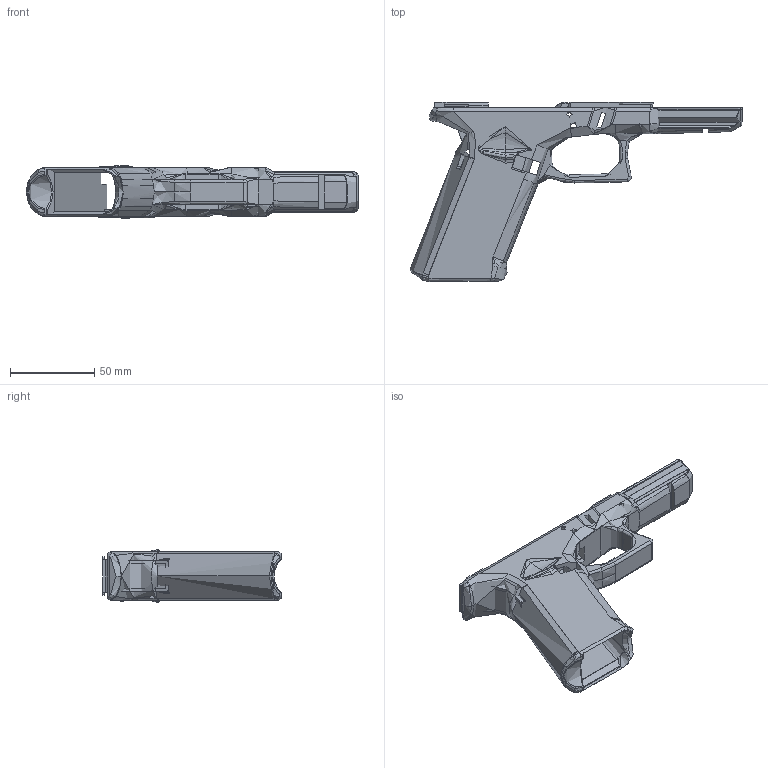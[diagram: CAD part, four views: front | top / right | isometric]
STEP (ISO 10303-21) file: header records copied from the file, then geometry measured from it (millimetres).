
FILE_DESCRIPTION(/* description */ (''),/* implementation_level */ '2;1');
FILE_NAME(/* name */ 'G17 P80 Rails.step',/* time_stamp */ '2019-09-29T13:28:27-04:00',/* author */ (''),/* organization */ (''),/* preprocessor_version */ 'ST-DEVELOPER v18',/* originating_system */ 'Autodesk Translation Framework v8.6.0.1094',/* authorisation */ '');
FILE_SCHEMA (('AUTOMOTIVE_DESIGN { 1 0 10303 214 3 1 1 }'));
Products named in the file (3): G17 P80 Rails; P80 Front Rails; P80 Rear Rails
Assembly tree (2 placements, depth 2):
  G17 P80 Rails
    P80 Front Rails
    P80 Rear Rails
Bounding box: 197.56 x 106.5 x 31.38 mm (x, y, z)
Volume: 94360.8 mm3
Topology: 3 solids, 7 shells, 878 faces, 2410 edges, 1509 vertices
Faces by surface type: bspline 382, plane 263, cylinder 183, torus 21, cone 19, sphere 10
Full cylindrical faces by diameter (mm): 3 x5, 3.2 x4, 3.5 x2, 3.8 x4
Entity records: 69030 total; most frequent: CARTESIAN_POINT 49261, ORIENTED_EDGE 4782, DIRECTION 3211, EDGE_CURVE 2391, VERTEX_POINT 1510, AXIS2_PLACEMENT_3D 1144, LINE 923, VECTOR 923
